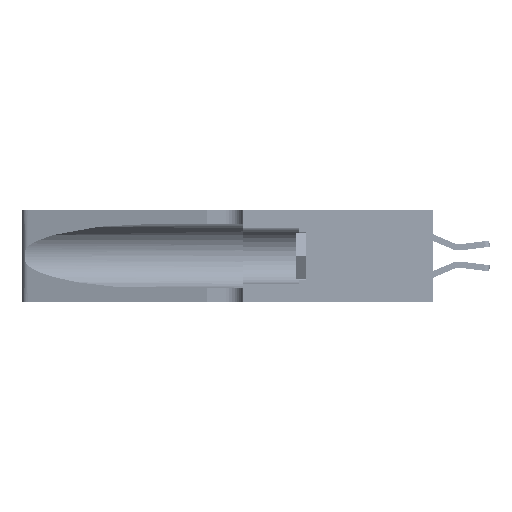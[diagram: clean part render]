
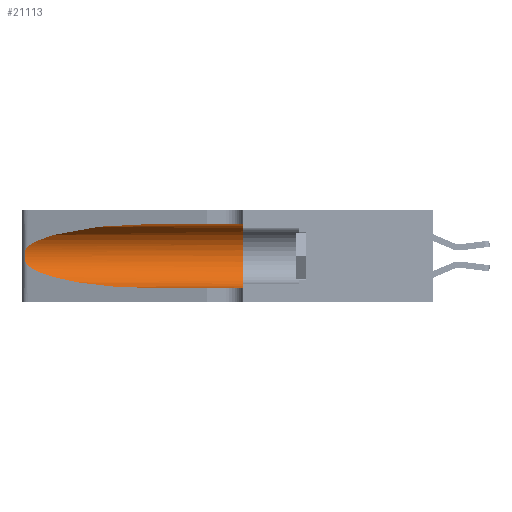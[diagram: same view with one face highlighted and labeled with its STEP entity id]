
A CAD part, left-side view. The second image highlights one B-rep face of the part: STEP entity #21113.
In plain terms, the highlighted cylindrical face has radius 3.308 mm (diameter 6.617 mm), a partial arc.
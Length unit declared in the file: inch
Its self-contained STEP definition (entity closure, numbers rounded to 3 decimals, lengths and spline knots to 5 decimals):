
#113 = ORIENTED_EDGE ( 'NONE', *, *, #28447, .F. ) ;
#254 = EDGE_CURVE ( 'NONE', #14411, #17204, #17438, .T. ) ;
#703 = FACE_OUTER_BOUND ( 'NONE', #38031, .T. ) ;
#1175 = CARTESIAN_POINT ( 'NONE',  ( 0.25555, 1.22993, 0.14849 ) ) ;
#1411 = VECTOR ( 'NONE', #15210, 39.37008 ) ;
#1566 = EDGE_CURVE ( 'NONE', #24295, #7122, #36161, .T. ) ;
#3428 = AXIS2_PLACEMENT_3D ( 'NONE', #12046, #32910, #15034 ) ;
#3433 = CARTESIAN_POINT ( 'NONE',  ( 0.1305, 1.61858, 0.185 ) ) ;
#4064 = CARTESIAN_POINT ( 'NONE',  ( 0.25487, 1.22718, 0.22369 ) ) ;
#4965 = VERTEX_POINT ( 'NONE', #13469 ) ;
#5501 = CIRCLE ( 'NONE', #3428, 0.13025 ) ;
#7093 = CARTESIAN_POINT ( 'NONE',  ( 0.25787, 1.23484, 0.2124 ) ) ;
#7122 = VERTEX_POINT ( 'NONE', #25209 ) ;
#8061 =( BOUNDED_CURVE ( )  B_SPLINE_CURVE ( 3, ( #10709, #28592, #34550, #16728 ),
 .UNSPECIFIED., .F., .T. ) 
 B_SPLINE_CURVE_WITH_KNOTS ( ( 4, 4 ),
 ( 1.5708, 2.84003 ),
 .UNSPECIFIED. ) 
 CURVE ( )  GEOMETRIC_REPRESENTATION_ITEM ( )  RATIONAL_B_SPLINE_CURVE ( ( 1., 0.87, 0.87, 1. ) ) 
 REPRESENTATION_ITEM ( '' )  );
#9530 = DIRECTION ( 'NONE',  ( 0., 0., -1. ) ) ;
#10162 = CARTESIAN_POINT ( 'NONE',  ( 0.26018, 1.23835, 0.19895 ) ) ;
#10545 = ORIENTED_EDGE ( 'NONE', *, *, #1566, .T. ) ;
#10709 = CARTESIAN_POINT ( 'NONE',  ( 0.1305, 0.72297, 0.31525 ) ) ;
#12046 = CARTESIAN_POINT ( 'NONE',  ( 0.1305, 0.35, 0.185 ) ) ;
#12794 = VECTOR ( 'NONE', #18109, 39.37008 ) ;
#12955 = CARTESIAN_POINT ( 'NONE',  ( 0.1305, 1.61858, 0.05475 ) ) ;
#13141 = CARTESIAN_POINT ( 'NONE',  ( 0.26075, 1.23896, 0.178 ) ) ;
#13469 = CARTESIAN_POINT ( 'NONE',  ( 0.1305, 0.35, 0.31525 ) ) ;
#14411 = VERTEX_POINT ( 'NONE', #29825 ) ;
#15034 = DIRECTION ( 'NONE',  ( 0., 0., 1. ) ) ;
#15210 = DIRECTION ( 'NONE',  ( 0., -1., 0. ) ) ;
#16188 = CARTESIAN_POINT ( 'NONE',  ( 0.25856, 1.23593, 0.16098 ) ) ;
#16250 = CARTESIAN_POINT ( 'NONE',  ( 0.2373, 1.15595, 0.08982 ) ) ;
#16728 = CARTESIAN_POINT ( 'NONE',  ( 0.25487, 1.22718, 0.22369 ) ) ;
#16740 = VERTEX_POINT ( 'NONE', #22011 ) ;
#17204 = VERTEX_POINT ( 'NONE', #27052 ) ;
#17438 = LINE ( 'NONE', #12955, #1411 ) ;
#18109 = DIRECTION ( 'NONE',  ( 0., -1., 0. ) ) ;
#19102 = CARTESIAN_POINT ( 'NONE',  ( 0.25555, 1.22994, 0.2215 ) ) ;
#19232 = CARTESIAN_POINT ( 'NONE',  ( 0.25639, 1.23186, 0.15144 ) ) ;
#19291 = CARTESIAN_POINT ( 'NONE',  ( 0.1305, 0.72297, 0.05475 ) ) ;
#20609 = EDGE_CURVE ( 'NONE', #7122, #14411, #33060, .T. ) ;
#21113 = ADVANCED_FACE ( 'NONE', ( #703 ), #38684, .F. ) ;
#21343 = ORIENTED_EDGE ( 'NONE', *, *, #32203, .F. ) ;
#22011 = CARTESIAN_POINT ( 'NONE',  ( 0.1305, 0.72297, 0.31525 ) ) ;
#22234 = CARTESIAN_POINT ( 'NONE',  ( 0.25487, 1.22718, 0.14631 ) ) ;
#24295 = VERTEX_POINT ( 'NONE', #28001 ) ;
#25109 = CARTESIAN_POINT ( 'NONE',  ( 0.25639, 1.23184, 0.21858 ) ) ;
#25209 = CARTESIAN_POINT ( 'NONE',  ( 0.25487, 1.22718, 0.14631 ) ) ;
#26476 = ORIENTED_EDGE ( 'NONE', *, *, #20609, .T. ) ;
#27052 = CARTESIAN_POINT ( 'NONE',  ( 0.1305, 0.35, 0.05475 ) ) ;
#27452 = DIRECTION ( 'NONE',  ( 0., -1., 0. ) ) ;
#27780 = LINE ( 'NONE', #35926, #12794 ) ;
#27818 = EDGE_CURVE ( 'NONE', #16740, #24295, #8061, .T. ) ;
#28001 = CARTESIAN_POINT ( 'NONE',  ( 0.25487, 1.22718, 0.22369 ) ) ;
#28069 = CARTESIAN_POINT ( 'NONE',  ( 0.25854, 1.2359, 0.20912 ) ) ;
#28315 = ORIENTED_EDGE ( 'NONE', *, *, #254, .T. ) ;
#28447 = EDGE_CURVE ( 'NONE', #16740, #4965, #27780, .T. ) ;
#28592 = CARTESIAN_POINT ( 'NONE',  ( 0.18966, 0.96281, 0.31525 ) ) ;
#29825 = CARTESIAN_POINT ( 'NONE',  ( 0.1305, 0.72297, 0.05475 ) ) ;
#31056 = CARTESIAN_POINT ( 'NONE',  ( 0.26075, 1.23896, 0.19203 ) ) ;
#32203 = EDGE_CURVE ( 'NONE', #4965, #17204, #5501, .T. ) ;
#32910 = DIRECTION ( 'NONE',  ( 0., 1., 0. ) ) ;
#33060 =( BOUNDED_CURVE ( )  B_SPLINE_CURVE ( 3, ( #34090, #16250, #37126, #19291 ),
 .UNSPECIFIED., .F., .T. ) 
 B_SPLINE_CURVE_WITH_KNOTS ( ( 4, 4 ),
 ( 3.44316, 4.71239 ),
 .UNSPECIFIED. ) 
 CURVE ( )  GEOMETRIC_REPRESENTATION_ITEM ( )  RATIONAL_B_SPLINE_CURVE ( ( 1., 0.87, 0.87, 1. ) ) 
 REPRESENTATION_ITEM ( '' )  );
#33397 = ORIENTED_EDGE ( 'NONE', *, *, #27818, .T. ) ;
#34018 = CARTESIAN_POINT ( 'NONE',  ( 0.26017, 1.23833, 0.17102 ) ) ;
#34090 = CARTESIAN_POINT ( 'NONE',  ( 0.25487, 1.22718, 0.14631 ) ) ;
#34550 = CARTESIAN_POINT ( 'NONE',  ( 0.2373, 1.15595, 0.28018 ) ) ;
#35926 = CARTESIAN_POINT ( 'NONE',  ( 0.1305, 1.61858, 0.31525 ) ) ;
#36161 = B_SPLINE_CURVE_WITH_KNOTS ( 'NONE', 3,
 ( #4064, #19102, #25109, #7093, #28069, #10162, #31056, #13141, #34018, #16188, #37048, #19232, #1175, #22234 ),
 .UNSPECIFIED., .F., .F.,
 ( 4, 2, 2, 2, 2, 2, 4 ),
 ( 0., 0.00027, 0.00053, 0.00107, 0.0016, 0.00187, 0.00214 ),
 .UNSPECIFIED. ) ;
#37048 = CARTESIAN_POINT ( 'NONE',  ( 0.25789, 1.23486, 0.15765 ) ) ;
#37126 = CARTESIAN_POINT ( 'NONE',  ( 0.18966, 0.96281, 0.05475 ) ) ;
#37547 = AXIS2_PLACEMENT_3D ( 'NONE', #3433, #27452, #9530 ) ;
#38031 = EDGE_LOOP ( 'NONE', ( #33397, #10545, #26476, #28315, #21343, #113 ) ) ;
#38684 = CYLINDRICAL_SURFACE ( 'NONE', #37547, 0.13025 ) ;
